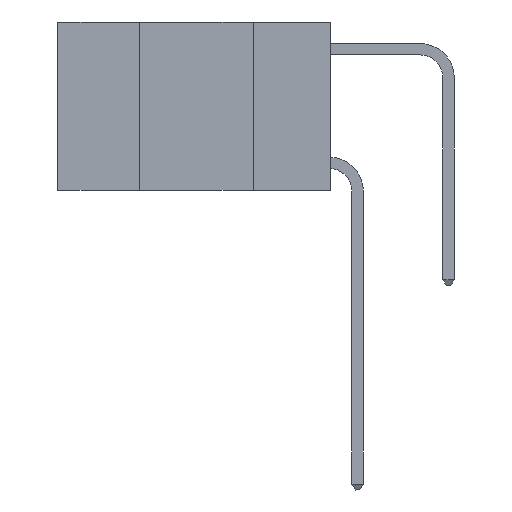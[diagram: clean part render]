
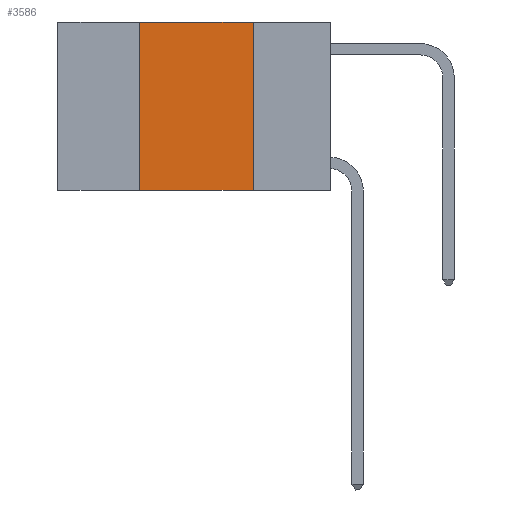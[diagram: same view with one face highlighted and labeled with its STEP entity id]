
A CAD part, left-side view. The second image highlights one B-rep face of the part: STEP entity #3586.
In plain terms, the highlighted planar face has unit normal (-1, 0, 0).
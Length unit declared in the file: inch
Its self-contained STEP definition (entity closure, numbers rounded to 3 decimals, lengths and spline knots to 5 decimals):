
#441 = DIRECTION ( 'NONE',  ( 0., 0., -1. ) ) ;
#619 = VERTEX_POINT ( 'NONE', #14719 ) ;
#1289 = CARTESIAN_POINT ( 'NONE',  ( 0., 0.6, -0.37 ) ) ;
#1355 = VECTOR ( 'NONE', #441, 39.37008 ) ;
#2544 = AXIS2_PLACEMENT_3D ( 'NONE', #7197, #4922, #7346 ) ;
#3309 = VERTEX_POINT ( 'NONE', #13581 ) ;
#3524 = VECTOR ( 'NONE', #5862, 39.37008 ) ;
#3586 = ADVANCED_FACE ( 'NONE', ( #8315 ), #11907, .F. ) ;
#3755 = DIRECTION ( 'NONE',  ( 0., -1., 0. ) ) ;
#3829 = CARTESIAN_POINT ( 'NONE',  ( 0., 0.6, 0. ) ) ;
#3830 = CARTESIAN_POINT ( 'NONE',  ( 0., 0.42, 0. ) ) ;
#4159 = ORIENTED_EDGE ( 'NONE', *, *, #12410, .F. ) ;
#4860 = LINE ( 'NONE', #8101, #13994 ) ;
#4922 = DIRECTION ( 'NONE',  ( 1., 0., 0. ) ) ;
#5862 = DIRECTION ( 'NONE',  ( 0., -1., 0. ) ) ;
#6876 = ORIENTED_EDGE ( 'NONE', *, *, #11050, .F. ) ;
#7197 = CARTESIAN_POINT ( 'NONE',  ( 0., 0.6, 0. ) ) ;
#7346 = DIRECTION ( 'NONE',  ( 0., 0., -1. ) ) ;
#8101 = CARTESIAN_POINT ( 'NONE',  ( 0., 0.42, 0. ) ) ;
#8119 = LINE ( 'NONE', #3829, #12985 ) ;
#8315 = FACE_OUTER_BOUND ( 'NONE', #8588, .T. ) ;
#8519 = EDGE_CURVE ( 'NONE', #12084, #11989, #8119, .T. ) ;
#8588 = EDGE_LOOP ( 'NONE', ( #6876, #9438, #4159, #9630 ) ) ;
#8822 = CARTESIAN_POINT ( 'NONE',  ( 0., 0.17, 0. ) ) ;
#9149 = CARTESIAN_POINT ( 'NONE',  ( 0., 0.17, 0. ) ) ;
#9438 = ORIENTED_EDGE ( 'NONE', *, *, #8519, .F. ) ;
#9630 = ORIENTED_EDGE ( 'NONE', *, *, #12007, .T. ) ;
#11050 = EDGE_CURVE ( 'NONE', #11989, #619, #12132, .T. ) ;
#11493 = LINE ( 'NONE', #1289, #3524 ) ;
#11907 = PLANE ( 'NONE',  #2544 ) ;
#11989 = VERTEX_POINT ( 'NONE', #9149 ) ;
#12007 = EDGE_CURVE ( 'NONE', #3309, #619, #11493, .T. ) ;
#12084 = VERTEX_POINT ( 'NONE', #3830 ) ;
#12132 = LINE ( 'NONE', #8822, #1355 ) ;
#12410 = EDGE_CURVE ( 'NONE', #3309, #12084, #4860, .T. ) ;
#12617 = DIRECTION ( 'NONE',  ( 0., 0., 1. ) ) ;
#12985 = VECTOR ( 'NONE', #3755, 39.37008 ) ;
#13581 = CARTESIAN_POINT ( 'NONE',  ( 0., 0.42, -0.37 ) ) ;
#13994 = VECTOR ( 'NONE', #12617, 39.37008 ) ;
#14719 = CARTESIAN_POINT ( 'NONE',  ( 0., 0.17, -0.37 ) ) ;
